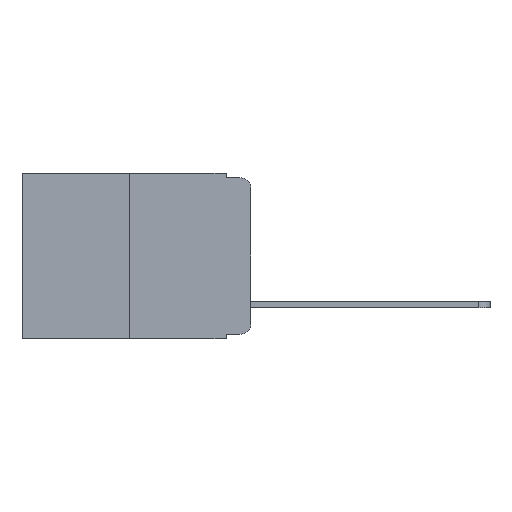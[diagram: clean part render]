
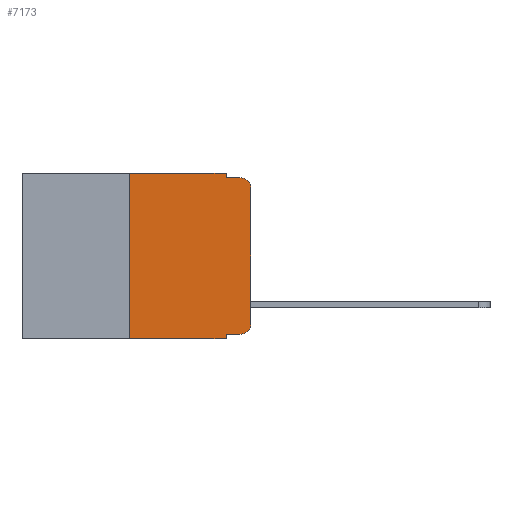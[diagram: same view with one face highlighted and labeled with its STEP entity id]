
A CAD part, left-side view. The second image highlights one B-rep face of the part: STEP entity #7173.
In plain terms, the highlighted planar face has unit normal (-1, 0, 0).
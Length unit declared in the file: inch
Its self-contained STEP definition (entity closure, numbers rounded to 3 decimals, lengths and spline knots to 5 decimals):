
#187 = EDGE_CURVE ( 'NONE', #13665, #13653, #4311, .T. ) ;
#381 = VERTEX_POINT ( 'NONE', #20362 ) ;
#396 = DIRECTION ( 'NONE',  ( 0., 0., -1. ) ) ;
#476 = DIRECTION ( 'NONE',  ( 0., 0., -1. ) ) ;
#805 = CARTESIAN_POINT ( 'NONE',  ( 0., 0., -0.03 ) ) ;
#1352 = ORIENTED_EDGE ( 'NONE', *, *, #19005, .T. ) ;
#1746 = CARTESIAN_POINT ( 'NONE',  ( 0., 0.051, -0.01 ) ) ;
#2190 = CARTESIAN_POINT ( 'NONE',  ( 0., 0.051, -0.333 ) ) ;
#2352 = VERTEX_POINT ( 'NONE', #12907 ) ;
#3207 = AXIS2_PLACEMENT_3D ( 'NONE', #20154, #18376, #7696 ) ;
#3670 = EDGE_CURVE ( 'NONE', #5512, #6232, #13516, .T. ) ;
#4056 = ORIENTED_EDGE ( 'NONE', *, *, #3670, .F. ) ;
#4168 = CARTESIAN_POINT ( 'NONE',  ( 0., 0.051, 0. ) ) ;
#4203 = LINE ( 'NONE', #4168, #22432 ) ;
#4244 = ORIENTED_EDGE ( 'NONE', *, *, #7879, .T. ) ;
#4311 = LINE ( 'NONE', #1746, #12150 ) ;
#4510 = EDGE_CURVE ( 'NONE', #10161, #13653, #19620, .T. ) ;
#4518 = CARTESIAN_POINT ( 'NONE',  ( 0., 0., 0. ) ) ;
#4658 = DIRECTION ( 'NONE',  ( 0., 0., -1. ) ) ;
#4937 = EDGE_CURVE ( 'NONE', #8228, #13665, #4203, .T. ) ;
#5016 = EDGE_CURVE ( 'NONE', #5418, #9436, #9231, .T. ) ;
#5241 = CARTESIAN_POINT ( 'NONE',  ( 0., 0.02, -0.333 ) ) ;
#5418 = VERTEX_POINT ( 'NONE', #5241 ) ;
#5512 = VERTEX_POINT ( 'NONE', #2190 ) ;
#5628 = CARTESIAN_POINT ( 'NONE',  ( 0., 0.051, 0. ) ) ;
#5906 = CARTESIAN_POINT ( 'NONE',  ( 0., 0.051, 0. ) ) ;
#6232 = VERTEX_POINT ( 'NONE', #19186 ) ;
#6460 = CARTESIAN_POINT ( 'NONE',  ( 0., 0.051, -0.333 ) ) ;
#6762 = AXIS2_PLACEMENT_3D ( 'NONE', #13872, #11941, #4658 ) ;
#7065 = EDGE_CURVE ( 'NONE', #2352, #381, #7270, .T. ) ;
#7173 = ADVANCED_FACE ( 'NONE', ( #17118 ), #14804, .F. ) ;
#7247 = DIRECTION ( 'NONE',  ( 0., -1., 0. ) ) ;
#7270 = LINE ( 'NONE', #12947, #17377 ) ;
#7595 = EDGE_CURVE ( 'NONE', #381, #8228, #16493, .T. ) ;
#7648 = DIRECTION ( 'NONE',  ( 0., -1., 0. ) ) ;
#7696 = DIRECTION ( 'NONE',  ( 0., 0., -1. ) ) ;
#7879 = EDGE_CURVE ( 'NONE', #9436, #10161, #13935, .T. ) ;
#7965 = ORIENTED_EDGE ( 'NONE', *, *, #7065, .F. ) ;
#8195 = VECTOR ( 'NONE', #12812, 39.37008 ) ;
#8228 = VERTEX_POINT ( 'NONE', #5906 ) ;
#8385 = AXIS2_PLACEMENT_3D ( 'NONE', #9314, #16459, #396 ) ;
#8644 = VECTOR ( 'NONE', #7247, 39.37008 ) ;
#8919 = EDGE_CURVE ( 'NONE', #2352, #6232, #15589, .T. ) ;
#9231 = CIRCLE ( 'NONE', #8385, 0.02 ) ;
#9314 = CARTESIAN_POINT ( 'NONE',  ( 0., 0.02, -0.313 ) ) ;
#9436 = VERTEX_POINT ( 'NONE', #22134 ) ;
#9443 = CARTESIAN_POINT ( 'NONE',  ( 0., 0.473, -0.343 ) ) ;
#10026 = DIRECTION ( 'NONE',  ( 0., -1., 0. ) ) ;
#10027 = VECTOR ( 'NONE', #13647, 39.37008 ) ;
#10161 = VERTEX_POINT ( 'NONE', #805 ) ;
#10843 = EDGE_LOOP ( 'NONE', ( #4244, #11354, #15044, #13527, #15956, #7965, #21390, #4056, #1352, #17117 ) ) ;
#11084 = CARTESIAN_POINT ( 'NONE',  ( 0., 0.473, 0. ) ) ;
#11096 = VECTOR ( 'NONE', #7648, 39.37008 ) ;
#11354 = ORIENTED_EDGE ( 'NONE', *, *, #4510, .T. ) ;
#11941 = DIRECTION ( 'NONE',  ( -1., 0., 0. ) ) ;
#12150 = VECTOR ( 'NONE', #19650, 39.37008 ) ;
#12812 = DIRECTION ( 'NONE',  ( 0., 0., -1. ) ) ;
#12907 = CARTESIAN_POINT ( 'NONE',  ( 0., 0.25, -0.343 ) ) ;
#12947 = CARTESIAN_POINT ( 'NONE',  ( 0., 0.25, 0. ) ) ;
#13516 = LINE ( 'NONE', #5628, #8195 ) ;
#13527 = ORIENTED_EDGE ( 'NONE', *, *, #4937, .F. ) ;
#13647 = DIRECTION ( 'NONE',  ( 0., 0., 1. ) ) ;
#13653 = VERTEX_POINT ( 'NONE', #22625 ) ;
#13665 = VERTEX_POINT ( 'NONE', #17154 ) ;
#13872 = CARTESIAN_POINT ( 'NONE',  ( 0., 0.02, -0.03 ) ) ;
#13935 = LINE ( 'NONE', #4518, #10027 ) ;
#14804 = PLANE ( 'NONE',  #3207 ) ;
#15044 = ORIENTED_EDGE ( 'NONE', *, *, #187, .F. ) ;
#15589 = LINE ( 'NONE', #9443, #11096 ) ;
#15956 = ORIENTED_EDGE ( 'NONE', *, *, #7595, .F. ) ;
#16459 = DIRECTION ( 'NONE',  ( -1., 0., 0. ) ) ;
#16493 = LINE ( 'NONE', #11084, #8644 ) ;
#17117 = ORIENTED_EDGE ( 'NONE', *, *, #5016, .T. ) ;
#17118 = FACE_OUTER_BOUND ( 'NONE', #10843, .T. ) ;
#17154 = CARTESIAN_POINT ( 'NONE',  ( 0., 0.051, -0.01 ) ) ;
#17377 = VECTOR ( 'NONE', #18056, 39.37008 ) ;
#17402 = VECTOR ( 'NONE', #10026, 39.37008 ) ;
#18056 = DIRECTION ( 'NONE',  ( 0., 0., 1. ) ) ;
#18376 = DIRECTION ( 'NONE',  ( 1., 0., 0. ) ) ;
#19005 = EDGE_CURVE ( 'NONE', #5512, #5418, #21329, .T. ) ;
#19186 = CARTESIAN_POINT ( 'NONE',  ( 0., 0.051, -0.343 ) ) ;
#19620 = CIRCLE ( 'NONE', #6762, 0.02 ) ;
#19650 = DIRECTION ( 'NONE',  ( 0., -1., 0. ) ) ;
#20154 = CARTESIAN_POINT ( 'NONE',  ( 0., 0.473, 0. ) ) ;
#20362 = CARTESIAN_POINT ( 'NONE',  ( 0., 0.25, 0. ) ) ;
#21329 = LINE ( 'NONE', #6460, #17402 ) ;
#21390 = ORIENTED_EDGE ( 'NONE', *, *, #8919, .T. ) ;
#22134 = CARTESIAN_POINT ( 'NONE',  ( 0., 0., -0.313 ) ) ;
#22432 = VECTOR ( 'NONE', #476, 39.37008 ) ;
#22625 = CARTESIAN_POINT ( 'NONE',  ( 0., 0.02, -0.01 ) ) ;
